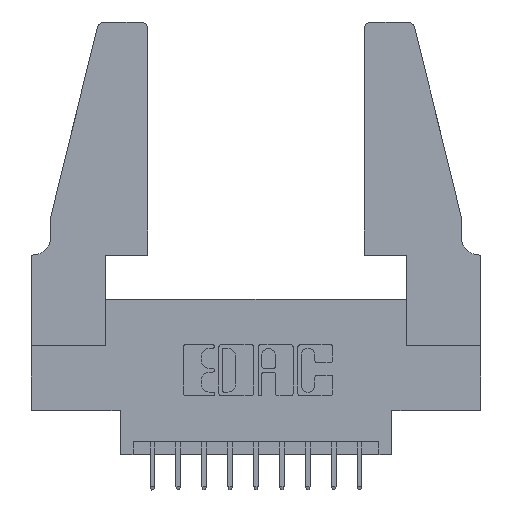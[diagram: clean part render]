
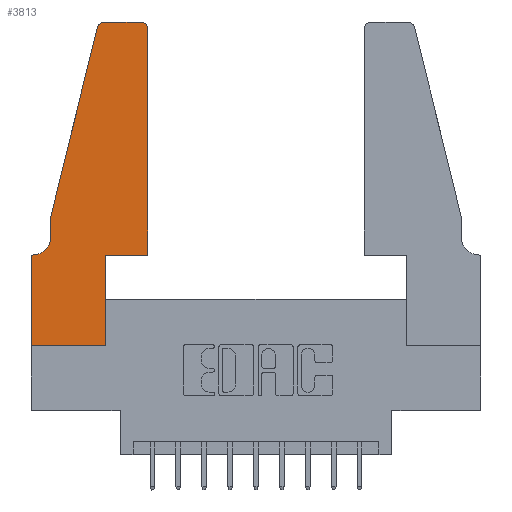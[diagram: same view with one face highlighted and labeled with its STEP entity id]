
A CAD part, top view. The second image highlights one B-rep face of the part: STEP entity #3813.
In plain terms, the highlighted planar face has unit normal (0, 0, 1).
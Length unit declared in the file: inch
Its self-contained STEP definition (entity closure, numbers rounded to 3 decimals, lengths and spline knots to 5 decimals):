
#78 = LINE ( 'NONE', #6469, #12005 ) ;
#191 = EDGE_CURVE ( 'NONE', #4766, #10485, #7753, .T. ) ;
#213 = CARTESIAN_POINT ( 'NONE',  ( 0.0055, 0.35, 0.37 ) ) ;
#371 = VERTEX_POINT ( 'NONE', #213 ) ;
#408 = LINE ( 'NONE', #4720, #11932 ) ;
#466 = EDGE_CURVE ( 'NONE', #3944, #1344, #11693, .T. ) ;
#538 = VERTEX_POINT ( 'NONE', #2683 ) ;
#557 = CARTESIAN_POINT ( 'NONE',  ( 0.2865, 0., 0.37 ) ) ;
#802 = EDGE_CURVE ( 'NONE', #371, #4766, #10877, .T. ) ;
#936 = DIRECTION ( 'NONE',  ( 0., 0., 1. ) ) ;
#1085 = CARTESIAN_POINT ( 'NONE',  ( 0., 0.35, 0.37 ) ) ;
#1115 = DIRECTION ( 'NONE',  ( 1., 0., 0. ) ) ;
#1344 = VERTEX_POINT ( 'NONE', #13468 ) ;
#1397 = ORIENTED_EDGE ( 'NONE', *, *, #8116, .T. ) ;
#1691 = VECTOR ( 'NONE', #12019, 39.37008 ) ;
#1809 = ORIENTED_EDGE ( 'NONE', *, *, #191, .T. ) ;
#1842 = VERTEX_POINT ( 'NONE', #9346 ) ;
#1848 = CARTESIAN_POINT ( 'NONE',  ( 0.2865, 0.35, 0.37 ) ) ;
#1987 = FACE_OUTER_BOUND ( 'NONE', #9515, .T. ) ;
#1997 = LINE ( 'NONE', #6348, #2552 ) ;
#2014 = DIRECTION ( 'NONE',  ( -1., 0., 0. ) ) ;
#2058 = DIRECTION ( 'NONE',  ( 0., 0., 1. ) ) ;
#2082 = ORIENTED_EDGE ( 'NONE', *, *, #10166, .T. ) ;
#2386 = DIRECTION ( 'NONE',  ( 0., -1., 0. ) ) ;
#2552 = VECTOR ( 'NONE', #13812, 39.37008 ) ;
#2683 = CARTESIAN_POINT ( 'NONE',  ( 0.4505, 1.22, 0.37 ) ) ;
#2736 = VERTEX_POINT ( 'NONE', #1848 ) ;
#3153 = EDGE_CURVE ( 'NONE', #9813, #2736, #78, .T. ) ;
#3154 = DIRECTION ( 'NONE',  ( 0., 0., -1. ) ) ;
#3170 = DIRECTION ( 'NONE',  ( 0., 1., 0. ) ) ;
#3194 = EDGE_CURVE ( 'NONE', #2736, #12852, #9727, .T. ) ;
#3249 = CARTESIAN_POINT ( 'NONE',  ( 0.4505, 0.35, 0.37 ) ) ;
#3518 = CARTESIAN_POINT ( 'NONE',  ( 0.0755, 0.35, 0.37 ) ) ;
#3783 = ORIENTED_EDGE ( 'NONE', *, *, #13684, .T. ) ;
#3813 = ADVANCED_FACE ( 'NONE', ( #1987 ), #9558, .T. ) ;
#3944 = VERTEX_POINT ( 'NONE', #9744 ) ;
#4091 = CARTESIAN_POINT ( 'NONE',  ( 0., 0., 0.37 ) ) ;
#4128 = DIRECTION ( 'NONE',  ( 1., 0., 0. ) ) ;
#4276 = ORIENTED_EDGE ( 'NONE', *, *, #4612, .T. ) ;
#4480 = CARTESIAN_POINT ( 'NONE',  ( 0., 0., 0.37 ) ) ;
#4612 = EDGE_CURVE ( 'NONE', #1842, #5403, #5730, .T. ) ;
#4720 = CARTESIAN_POINT ( 'NONE',  ( 0., 0., 0.37 ) ) ;
#4766 = VERTEX_POINT ( 'NONE', #1085 ) ;
#4825 = CIRCLE ( 'NONE', #11964, 0.07 ) ;
#5007 = DIRECTION ( 'NONE',  ( -0.239, -0.971, 0. ) ) ;
#5403 = VERTEX_POINT ( 'NONE', #13653 ) ;
#5542 = CARTESIAN_POINT ( 'NONE',  ( 0.4505, 0.35, 0.37 ) ) ;
#5583 = AXIS2_PLACEMENT_3D ( 'NONE', #13217, #11013, #12023 ) ;
#5730 = LINE ( 'NONE', #11004, #11255 ) ;
#5782 = EDGE_CURVE ( 'NONE', #5403, #371, #4825, .T. ) ;
#5877 = LINE ( 'NONE', #7780, #1691 ) ;
#6107 = EDGE_CURVE ( 'NONE', #10485, #9813, #408, .T. ) ;
#6348 = CARTESIAN_POINT ( 'NONE',  ( 0.4505, 0.35, 0.37 ) ) ;
#6469 = CARTESIAN_POINT ( 'NONE',  ( 0.2865, 0.35, 0.37 ) ) ;
#6826 = DIRECTION ( 'NONE',  ( 0., -1., 0. ) ) ;
#6981 = ORIENTED_EDGE ( 'NONE', *, *, #6107, .T. ) ;
#7002 = ORIENTED_EDGE ( 'NONE', *, *, #5782, .T. ) ;
#7186 = VERTEX_POINT ( 'NONE', #11506 ) ;
#7191 = LINE ( 'NONE', #8362, #10892 ) ;
#7753 = LINE ( 'NONE', #4480, #11918 ) ;
#7780 = CARTESIAN_POINT ( 'NONE',  ( 0.2605, 1.25, 0.37 ) ) ;
#8030 = VECTOR ( 'NONE', #1115, 39.37008 ) ;
#8116 = EDGE_CURVE ( 'NONE', #7186, #3944, #5877, .T. ) ;
#8362 = CARTESIAN_POINT ( 'NONE',  ( 0.0755, 0.5, 0.37 ) ) ;
#8402 = AXIS2_PLACEMENT_3D ( 'NONE', #10379, #2058, #4128 ) ;
#8407 = ORIENTED_EDGE ( 'NONE', *, *, #802, .T. ) ;
#9346 = CARTESIAN_POINT ( 'NONE',  ( 0.0755, 0.5, 0.37 ) ) ;
#9476 = ORIENTED_EDGE ( 'NONE', *, *, #3153, .T. ) ;
#9515 = EDGE_LOOP ( 'NONE', ( #1397, #13423, #3783, #4276, #7002, #8407, #1809, #6981, #9476, #12016, #2082, #12100 ) ) ;
#9558 = PLANE ( 'NONE',  #8402 ) ;
#9639 = EDGE_CURVE ( 'NONE', #538, #7186, #12068, .T. ) ;
#9727 = LINE ( 'NONE', #5542, #8030 ) ;
#9744 = CARTESIAN_POINT ( 'NONE',  ( 0.284, 1.25, 0.37 ) ) ;
#9805 = DIRECTION ( 'NONE',  ( 1., 0., 0. ) ) ;
#9813 = VERTEX_POINT ( 'NONE', #557 ) ;
#10166 = EDGE_CURVE ( 'NONE', #12852, #538, #1997, .T. ) ;
#10379 = CARTESIAN_POINT ( 'NONE',  ( 0., 0.35, 0.37 ) ) ;
#10485 = VERTEX_POINT ( 'NONE', #4091 ) ;
#10489 = CARTESIAN_POINT ( 'NONE',  ( 0.0055, 0.42, 0.37 ) ) ;
#10575 = CARTESIAN_POINT ( 'NONE',  ( 0.284, 1.22, 0.37 ) ) ;
#10877 = LINE ( 'NONE', #3518, #13274 ) ;
#10892 = VECTOR ( 'NONE', #5007, 39.37008 ) ;
#11004 = CARTESIAN_POINT ( 'NONE',  ( 0.0755, 0.5, 0.37 ) ) ;
#11013 = DIRECTION ( 'NONE',  ( 0., 0., 1. ) ) ;
#11255 = VECTOR ( 'NONE', #2386, 39.37008 ) ;
#11506 = CARTESIAN_POINT ( 'NONE',  ( 0.4205, 1.25, 0.37 ) ) ;
#11693 = CIRCLE ( 'NONE', #13497, 0.03 ) ;
#11918 = VECTOR ( 'NONE', #6826, 39.37008 ) ;
#11932 = VECTOR ( 'NONE', #13346, 39.37008 ) ;
#11964 = AXIS2_PLACEMENT_3D ( 'NONE', #10489, #3154, #2014 ) ;
#12005 = VECTOR ( 'NONE', #3170, 39.37008 ) ;
#12012 = DIRECTION ( 'NONE',  ( -1., 0., 0. ) ) ;
#12016 = ORIENTED_EDGE ( 'NONE', *, *, #3194, .T. ) ;
#12019 = DIRECTION ( 'NONE',  ( -1., 0., 0. ) ) ;
#12023 = DIRECTION ( 'NONE',  ( 1., 0., 0. ) ) ;
#12068 = CIRCLE ( 'NONE', #5583, 0.03 ) ;
#12100 = ORIENTED_EDGE ( 'NONE', *, *, #9639, .T. ) ;
#12852 = VERTEX_POINT ( 'NONE', #3249 ) ;
#13217 = CARTESIAN_POINT ( 'NONE',  ( 0.4205, 1.22, 0.37 ) ) ;
#13274 = VECTOR ( 'NONE', #12012, 39.37008 ) ;
#13346 = DIRECTION ( 'NONE',  ( 1., 0., 0. ) ) ;
#13423 = ORIENTED_EDGE ( 'NONE', *, *, #466, .T. ) ;
#13468 = CARTESIAN_POINT ( 'NONE',  ( 0.25487, 1.22718, 0.37 ) ) ;
#13497 = AXIS2_PLACEMENT_3D ( 'NONE', #10575, #936, #9805 ) ;
#13653 = CARTESIAN_POINT ( 'NONE',  ( 0.0755, 0.42, 0.37 ) ) ;
#13684 = EDGE_CURVE ( 'NONE', #1344, #1842, #7191, .T. ) ;
#13812 = DIRECTION ( 'NONE',  ( 0., 1., 0. ) ) ;
